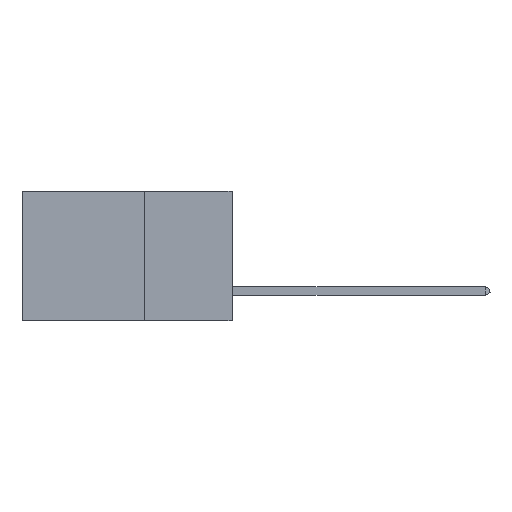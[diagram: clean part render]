
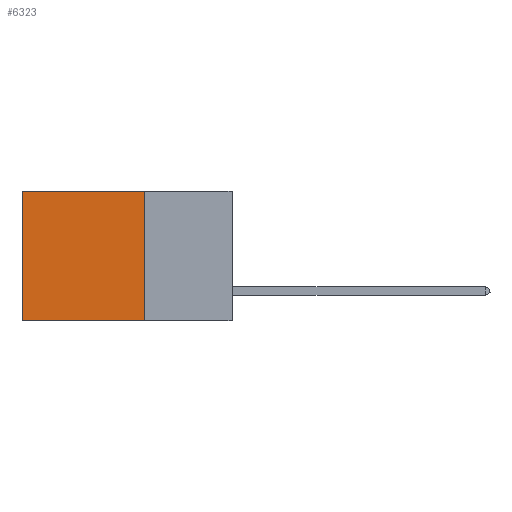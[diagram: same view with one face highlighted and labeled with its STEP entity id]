
A CAD part, left-side view. The second image highlights one B-rep face of the part: STEP entity #6323.
In plain terms, the highlighted planar face has unit normal (-1, 0, 0).
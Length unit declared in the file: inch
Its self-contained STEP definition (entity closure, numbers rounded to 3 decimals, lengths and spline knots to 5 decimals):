
#43 = FACE_OUTER_BOUND ( 'NONE', #4290, .T. ) ;
#739 = EDGE_CURVE ( 'NONE', #3551, #2500, #9683, .T. ) ;
#852 = VECTOR ( 'NONE', #10524, 39.37008 ) ;
#1048 = CARTESIAN_POINT ( 'NONE',  ( 0.2875, 0.6, 0. ) ) ;
#1881 = CARTESIAN_POINT ( 'NONE',  ( 0.2875, 0.25, -0.37 ) ) ;
#2500 = VERTEX_POINT ( 'NONE', #8890 ) ;
#3551 = VERTEX_POINT ( 'NONE', #1881 ) ;
#4054 = VECTOR ( 'NONE', #5587, 39.37008 ) ;
#4069 = LINE ( 'NONE', #13909, #852 ) ;
#4290 = EDGE_LOOP ( 'NONE', ( #6713, #13123, #10935, #5465 ) ) ;
#4678 = EDGE_CURVE ( 'NONE', #12332, #9717, #6719, .T. ) ;
#4724 = VECTOR ( 'NONE', #8125, 39.37008 ) ;
#4856 = DIRECTION ( 'NONE',  ( 1., 0., 0. ) ) ;
#5465 = ORIENTED_EDGE ( 'NONE', *, *, #4678, .T. ) ;
#5587 = DIRECTION ( 'NONE',  ( 0., 1., 0. ) ) ;
#5595 = CARTESIAN_POINT ( 'NONE',  ( 0.2875, 0.6, 0. ) ) ;
#5727 = CARTESIAN_POINT ( 'NONE',  ( 0.2875, 0.25, 0. ) ) ;
#6323 = ADVANCED_FACE ( 'NONE', ( #43 ), #7071, .F. ) ;
#6713 = ORIENTED_EDGE ( 'NONE', *, *, #9047, .T. ) ;
#6719 = LINE ( 'NONE', #5727, #12006 ) ;
#6932 = DIRECTION ( 'NONE',  ( 0., 1., 0. ) ) ;
#7071 = PLANE ( 'NONE',  #10219 ) ;
#7902 = LINE ( 'NONE', #1048, #4724 ) ;
#8125 = DIRECTION ( 'NONE',  ( 0., 0., -1. ) ) ;
#8314 = CARTESIAN_POINT ( 'NONE',  ( 0.2875, 0.25, 0. ) ) ;
#8890 = CARTESIAN_POINT ( 'NONE',  ( 0.2875, 0.6, -0.37 ) ) ;
#9047 = EDGE_CURVE ( 'NONE', #9717, #2500, #7902, .T. ) ;
#9683 = LINE ( 'NONE', #13409, #4054 ) ;
#9717 = VERTEX_POINT ( 'NONE', #5595 ) ;
#10219 = AXIS2_PLACEMENT_3D ( 'NONE', #10742, #4856, #11959 ) ;
#10524 = DIRECTION ( 'NONE',  ( 0., 0., -1. ) ) ;
#10742 = CARTESIAN_POINT ( 'NONE',  ( 0.2875, 0.25, 0. ) ) ;
#10935 = ORIENTED_EDGE ( 'NONE', *, *, #12005, .F. ) ;
#11959 = DIRECTION ( 'NONE',  ( 0., 0., -1. ) ) ;
#12005 = EDGE_CURVE ( 'NONE', #12332, #3551, #4069, .T. ) ;
#12006 = VECTOR ( 'NONE', #6932, 39.37008 ) ;
#12332 = VERTEX_POINT ( 'NONE', #8314 ) ;
#13123 = ORIENTED_EDGE ( 'NONE', *, *, #739, .F. ) ;
#13409 = CARTESIAN_POINT ( 'NONE',  ( 0.2875, 0.25, -0.37 ) ) ;
#13909 = CARTESIAN_POINT ( 'NONE',  ( 0.2875, 0.25, 0. ) ) ;
